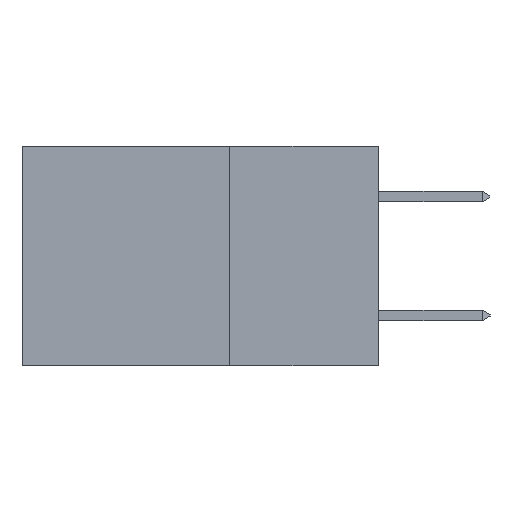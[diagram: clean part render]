
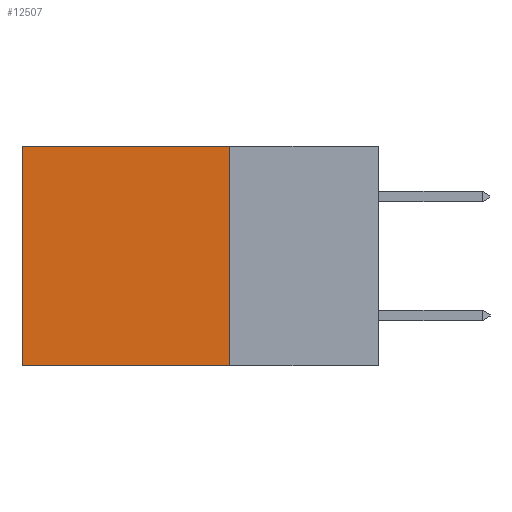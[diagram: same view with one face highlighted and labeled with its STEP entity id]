
A CAD part, left-side view. The second image highlights one B-rep face of the part: STEP entity #12507.
In plain terms, the highlighted planar face has unit normal (-1, 0, 0).
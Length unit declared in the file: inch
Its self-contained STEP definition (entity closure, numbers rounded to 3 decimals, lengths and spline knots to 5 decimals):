
#1060 = LINE ( 'NONE', #5842, #17560 ) ;
#1278 = EDGE_LOOP ( 'NONE', ( #6332, #18307, #6764, #9628 ) ) ;
#2286 = FACE_OUTER_BOUND ( 'NONE', #1278, .T. ) ;
#2319 = CARTESIAN_POINT ( 'NONE',  ( 0.2615, 0.25, -0.37 ) ) ;
#2898 = LINE ( 'NONE', #11193, #10873 ) ;
#4132 = CARTESIAN_POINT ( 'NONE',  ( 0.2615, 0.6, 0. ) ) ;
#5642 = VECTOR ( 'NONE', #12937, 39.37008 ) ;
#5842 = CARTESIAN_POINT ( 'NONE',  ( 0.2615, 0.25, 0. ) ) ;
#6106 = VECTOR ( 'NONE', #13536, 39.37008 ) ;
#6332 = ORIENTED_EDGE ( 'NONE', *, *, #15291, .T. ) ;
#6626 = LINE ( 'NONE', #8160, #5642 ) ;
#6764 = ORIENTED_EDGE ( 'NONE', *, *, #15234, .F. ) ;
#7549 = EDGE_CURVE ( 'NONE', #10694, #9671, #10844, .T. ) ;
#7567 = DIRECTION ( 'NONE',  ( 0., 0., -1. ) ) ;
#7803 = CARTESIAN_POINT ( 'NONE',  ( 0.2615, 0.6, -0.37 ) ) ;
#8160 = CARTESIAN_POINT ( 'NONE',  ( 0.2615, 0.6, -0.37 ) ) ;
#9024 = DIRECTION ( 'NONE',  ( 0., 1., 0. ) ) ;
#9244 = VERTEX_POINT ( 'NONE', #9987 ) ;
#9628 = ORIENTED_EDGE ( 'NONE', *, *, #16970, .T. ) ;
#9671 = VERTEX_POINT ( 'NONE', #7803 ) ;
#9987 = CARTESIAN_POINT ( 'NONE',  ( 0.2615, 0.25, 0. ) ) ;
#10694 = VERTEX_POINT ( 'NONE', #11704 ) ;
#10711 = PLANE ( 'NONE',  #11728 ) ;
#10844 = LINE ( 'NONE', #2319, #6106 ) ;
#10873 = VECTOR ( 'NONE', #17619, 39.37008 ) ;
#11193 = CARTESIAN_POINT ( 'NONE',  ( 0.2615, 0.25, -0.37 ) ) ;
#11704 = CARTESIAN_POINT ( 'NONE',  ( 0.2615, 0.25, -0.37 ) ) ;
#11728 = AXIS2_PLACEMENT_3D ( 'NONE', #15531, #17161, #7567 ) ;
#12507 = ADVANCED_FACE ( 'NONE', ( #2286 ), #10711, .F. ) ;
#12937 = DIRECTION ( 'NONE',  ( 0., 0., -1. ) ) ;
#13536 = DIRECTION ( 'NONE',  ( 0., 1., 0. ) ) ;
#15234 = EDGE_CURVE ( 'NONE', #9244, #10694, #2898, .T. ) ;
#15291 = EDGE_CURVE ( 'NONE', #18291, #9671, #6626, .T. ) ;
#15531 = CARTESIAN_POINT ( 'NONE',  ( 0.2615, 0.25, -0.37 ) ) ;
#16970 = EDGE_CURVE ( 'NONE', #9244, #18291, #1060, .T. ) ;
#17161 = DIRECTION ( 'NONE',  ( 1., 0., 0. ) ) ;
#17560 = VECTOR ( 'NONE', #9024, 39.37008 ) ;
#17619 = DIRECTION ( 'NONE',  ( 0., 0., -1. ) ) ;
#18291 = VERTEX_POINT ( 'NONE', #4132 ) ;
#18307 = ORIENTED_EDGE ( 'NONE', *, *, #7549, .F. ) ;
